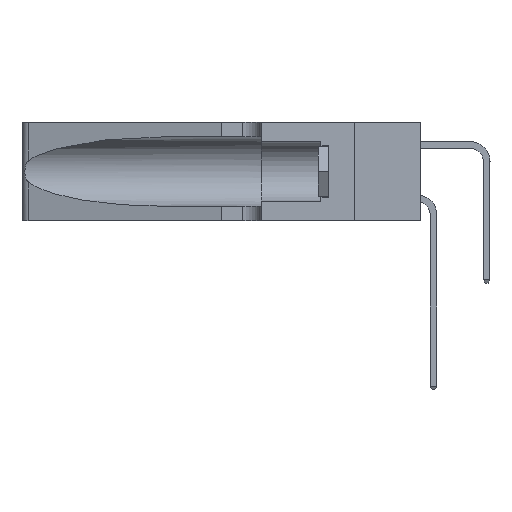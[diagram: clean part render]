
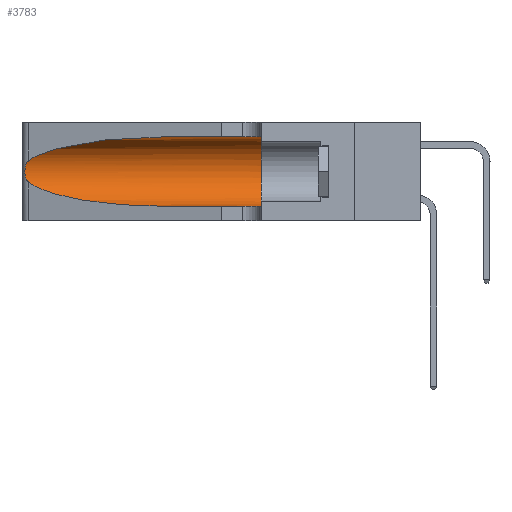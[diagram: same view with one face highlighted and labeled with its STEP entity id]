
A CAD part, left-side view. The second image highlights one B-rep face of the part: STEP entity #3783.
In plain terms, the highlighted cylindrical face has radius 3.308 mm (diameter 6.617 mm), a partial arc.
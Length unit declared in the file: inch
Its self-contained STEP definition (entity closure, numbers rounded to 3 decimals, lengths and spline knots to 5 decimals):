
#116 = CARTESIAN_POINT ( 'NONE',  ( 0.25639, 1.23186, 0.15144 ) ) ;
#196 = CARTESIAN_POINT ( 'NONE',  ( 0.25856, 1.23593, 0.16098 ) ) ;
#318 = CARTESIAN_POINT ( 'NONE',  ( 0.25555, 1.22993, 0.14849 ) ) ;
#504 = CARTESIAN_POINT ( 'NONE',  ( 0.26017, 1.23833, 0.17102 ) ) ;
#603 = VERTEX_POINT ( 'NONE', #24356 ) ;
#1150 = FACE_OUTER_BOUND ( 'NONE', #30611, .T. ) ;
#1603 = LINE ( 'NONE', #17054, #1986 ) ;
#1986 = VECTOR ( 'NONE', #2469, 39.37008 ) ;
#2397 = CARTESIAN_POINT ( 'NONE',  ( 0.1305, 1.61858, 0.05475 ) ) ;
#2469 = DIRECTION ( 'NONE',  ( 0., -1., 0. ) ) ;
#3284 = VERTEX_POINT ( 'NONE', #29394 ) ;
#3303 = B_SPLINE_CURVE_WITH_KNOTS ( 'NONE', 3,
 ( #6086, #24536, #32219, #19893, #31998, #17173, #25364, #30123, #504, #196, #27637, #116, #318, #20113 ),
 .UNSPECIFIED., .F., .F.,
 ( 4, 2, 2, 2, 2, 2, 4 ),
 ( 0., 0.00027, 0.00053, 0.00107, 0.0016, 0.00187, 0.00214 ),
 .UNSPECIFIED. ) ;
#3411 = CARTESIAN_POINT ( 'NONE',  ( 0.1305, 0.35, 0.05475 ) ) ;
#3783 = ADVANCED_FACE ( 'NONE', ( #1150 ), #4647, .F. ) ;
#4647 = CYLINDRICAL_SURFACE ( 'NONE', #24500, 0.13025 ) ;
#4957 = CARTESIAN_POINT ( 'NONE',  ( 0.1305, 0.72297, 0.31525 ) ) ;
#6086 = CARTESIAN_POINT ( 'NONE',  ( 0.25487, 1.22718, 0.22369 ) ) ;
#6585 = EDGE_CURVE ( 'NONE', #603, #3284, #3303, .T. ) ;
#6745 = DIRECTION ( 'NONE',  ( 0., -1., 0. ) ) ;
#6859 = CARTESIAN_POINT ( 'NONE',  ( 0.1305, 1.61858, 0.185 ) ) ;
#7380 = CARTESIAN_POINT ( 'NONE',  ( 0.1305, 0.72297, 0.31525 ) ) ;
#7396 = CARTESIAN_POINT ( 'NONE',  ( 0.1305, 0.35, 0.185 ) ) ;
#8442 = AXIS2_PLACEMENT_3D ( 'NONE', #7396, #32210, #19674 ) ;
#8608 = EDGE_CURVE ( 'NONE', #29105, #12609, #28874, .T. ) ;
#9012 = VECTOR ( 'NONE', #15750, 39.37008 ) ;
#9234 = DIRECTION ( 'NONE',  ( 0., 0., -1. ) ) ;
#10059 = ORIENTED_EDGE ( 'NONE', *, *, #29017, .T. ) ;
#10989 = ORIENTED_EDGE ( 'NONE', *, *, #31876, .F. ) ;
#12609 = VERTEX_POINT ( 'NONE', #3411 ) ;
#12805 = ORIENTED_EDGE ( 'NONE', *, *, #6585, .T. ) ;
#12894 = CARTESIAN_POINT ( 'NONE',  ( 0.1305, 0.72297, 0.05475 ) ) ;
#15750 = DIRECTION ( 'NONE',  ( 0., -1., 0. ) ) ;
#17054 = CARTESIAN_POINT ( 'NONE',  ( 0.1305, 1.61858, 0.31525 ) ) ;
#17156 = CARTESIAN_POINT ( 'NONE',  ( 0.25487, 1.22718, 0.22369 ) ) ;
#17173 = CARTESIAN_POINT ( 'NONE',  ( 0.26018, 1.23835, 0.19895 ) ) ;
#18042 = VERTEX_POINT ( 'NONE', #7380 ) ;
#19674 = DIRECTION ( 'NONE',  ( 0., 0., 1. ) ) ;
#19893 = CARTESIAN_POINT ( 'NONE',  ( 0.25787, 1.23484, 0.2124 ) ) ;
#20113 = CARTESIAN_POINT ( 'NONE',  ( 0.25487, 1.22718, 0.14631 ) ) ;
#20377 = CARTESIAN_POINT ( 'NONE',  ( 0.2373, 1.15595, 0.08982 ) ) ;
#21969 = EDGE_CURVE ( 'NONE', #3284, #29105, #27480, .T. ) ;
#22635 = ORIENTED_EDGE ( 'NONE', *, *, #8608, .T. ) ;
#22922 = CARTESIAN_POINT ( 'NONE',  ( 0.1305, 0.72297, 0.05475 ) ) ;
#23080 = VERTEX_POINT ( 'NONE', #30471 ) ;
#24212 = CIRCLE ( 'NONE', #8442, 0.13025 ) ;
#24356 = CARTESIAN_POINT ( 'NONE',  ( 0.25487, 1.22718, 0.22369 ) ) ;
#24500 = AXIS2_PLACEMENT_3D ( 'NONE', #6859, #6745, #9234 ) ;
#24536 = CARTESIAN_POINT ( 'NONE',  ( 0.25555, 1.22994, 0.2215 ) ) ;
#24711 = CARTESIAN_POINT ( 'NONE',  ( 0.2373, 1.15595, 0.28018 ) ) ;
#25095 =( BOUNDED_CURVE ( )  B_SPLINE_CURVE ( 3, ( #4957, #29490, #24711, #17156 ),
 .UNSPECIFIED., .F., .T. ) 
 B_SPLINE_CURVE_WITH_KNOTS ( ( 4, 4 ),
 ( 1.5708, 2.84003 ),
 .UNSPECIFIED. ) 
 CURVE ( )  GEOMETRIC_REPRESENTATION_ITEM ( )  RATIONAL_B_SPLINE_CURVE ( ( 1., 0.87, 0.87, 1. ) ) 
 REPRESENTATION_ITEM ( '' )  );
#25364 = CARTESIAN_POINT ( 'NONE',  ( 0.26075, 1.23896, 0.19203 ) ) ;
#27033 = ORIENTED_EDGE ( 'NONE', *, *, #31846, .F. ) ;
#27480 =( BOUNDED_CURVE ( )  B_SPLINE_CURVE ( 3, ( #30089, #20377, #28042, #22922 ),
 .UNSPECIFIED., .F., .T. ) 
 B_SPLINE_CURVE_WITH_KNOTS ( ( 4, 4 ),
 ( 3.44316, 4.71239 ),
 .UNSPECIFIED. ) 
 CURVE ( )  GEOMETRIC_REPRESENTATION_ITEM ( )  RATIONAL_B_SPLINE_CURVE ( ( 1., 0.87, 0.87, 1. ) ) 
 REPRESENTATION_ITEM ( '' )  );
#27637 = CARTESIAN_POINT ( 'NONE',  ( 0.25789, 1.23486, 0.15765 ) ) ;
#28042 = CARTESIAN_POINT ( 'NONE',  ( 0.18966, 0.96281, 0.05475 ) ) ;
#28874 = LINE ( 'NONE', #2397, #9012 ) ;
#29017 = EDGE_CURVE ( 'NONE', #18042, #603, #25095, .T. ) ;
#29105 = VERTEX_POINT ( 'NONE', #12894 ) ;
#29394 = CARTESIAN_POINT ( 'NONE',  ( 0.25487, 1.22718, 0.14631 ) ) ;
#29490 = CARTESIAN_POINT ( 'NONE',  ( 0.18966, 0.96281, 0.31525 ) ) ;
#30089 = CARTESIAN_POINT ( 'NONE',  ( 0.25487, 1.22718, 0.14631 ) ) ;
#30123 = CARTESIAN_POINT ( 'NONE',  ( 0.26075, 1.23896, 0.178 ) ) ;
#30471 = CARTESIAN_POINT ( 'NONE',  ( 0.1305, 0.35, 0.31525 ) ) ;
#30611 = EDGE_LOOP ( 'NONE', ( #10059, #12805, #32030, #22635, #27033, #10989 ) ) ;
#31846 = EDGE_CURVE ( 'NONE', #23080, #12609, #24212, .T. ) ;
#31876 = EDGE_CURVE ( 'NONE', #18042, #23080, #1603, .T. ) ;
#31998 = CARTESIAN_POINT ( 'NONE',  ( 0.25854, 1.2359, 0.20912 ) ) ;
#32030 = ORIENTED_EDGE ( 'NONE', *, *, #21969, .T. ) ;
#32210 = DIRECTION ( 'NONE',  ( 0., 1., 0. ) ) ;
#32219 = CARTESIAN_POINT ( 'NONE',  ( 0.25639, 1.23184, 0.21858 ) ) ;
